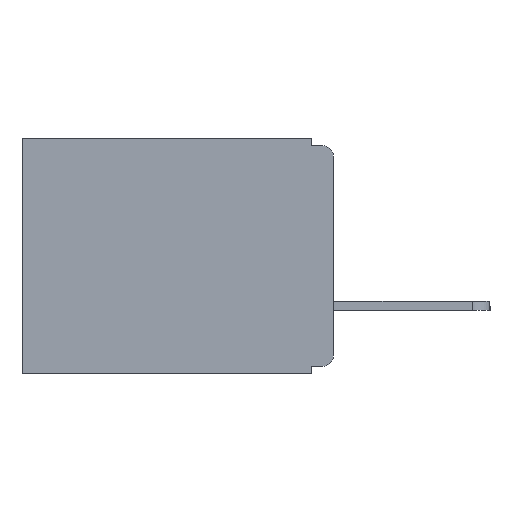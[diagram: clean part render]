
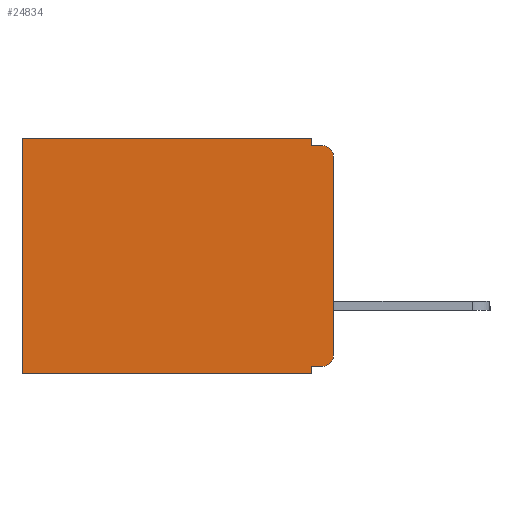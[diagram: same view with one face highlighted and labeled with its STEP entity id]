
A CAD part, left-side view. The second image highlights one B-rep face of the part: STEP entity #24834.
In plain terms, the highlighted planar face has unit normal (-1, 0, 0).
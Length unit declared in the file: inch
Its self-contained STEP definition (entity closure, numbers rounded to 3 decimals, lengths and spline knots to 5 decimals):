
#348 = EDGE_LOOP ( 'NONE', ( #8116, #9659, #23048, #16665, #27672, #12889, #12502, #18715, #5621, #6374 ) ) ;
#965 = EDGE_CURVE ( 'NONE', #14037, #2807, #26319, .T. ) ;
#1911 = VERTEX_POINT ( 'NONE', #20017 ) ;
#2025 = CARTESIAN_POINT ( 'NONE',  ( 0.3, 0.031, 0. ) ) ;
#2807 = VERTEX_POINT ( 'NONE', #31010 ) ;
#3529 = LINE ( 'NONE', #29096, #9255 ) ;
#3638 = VECTOR ( 'NONE', #30112, 39.37008 ) ;
#3853 = VECTOR ( 'NONE', #30522, 39.37008 ) ;
#4380 = EDGE_CURVE ( 'NONE', #2807, #25209, #14804, .T. ) ;
#4521 = DIRECTION ( 'NONE',  ( 1., 0., 0. ) ) ;
#5217 = CARTESIAN_POINT ( 'NONE',  ( 0.3, 0., -0.025 ) ) ;
#5401 = CARTESIAN_POINT ( 'NONE',  ( 0.3, 0., -0.32 ) ) ;
#5452 = EDGE_CURVE ( 'NONE', #5602, #23584, #20508, .T. ) ;
#5579 = EDGE_CURVE ( 'NONE', #1911, #7438, #26923, .T. ) ;
#5602 = VERTEX_POINT ( 'NONE', #27760 ) ;
#5621 = ORIENTED_EDGE ( 'NONE', *, *, #24429, .F. ) ;
#5715 = AXIS2_PLACEMENT_3D ( 'NONE', #19212, #4521, #21662 ) ;
#6340 = CARTESIAN_POINT ( 'NONE',  ( 0.3, 0., -0.33 ) ) ;
#6374 = ORIENTED_EDGE ( 'NONE', *, *, #7396, .T. ) ;
#6567 = CIRCLE ( 'NONE', #19662, 0.015 ) ;
#6825 = VECTOR ( 'NONE', #17000, 39.37008 ) ;
#7396 = EDGE_CURVE ( 'NONE', #10517, #30683, #16577, .T. ) ;
#7438 = VERTEX_POINT ( 'NONE', #13631 ) ;
#7492 = VECTOR ( 'NONE', #14709, 39.37008 ) ;
#7921 = LINE ( 'NONE', #5401, #13666 ) ;
#8116 = ORIENTED_EDGE ( 'NONE', *, *, #12113, .F. ) ;
#8839 = DIRECTION ( 'NONE',  ( 0., 0., -1. ) ) ;
#9255 = VECTOR ( 'NONE', #9646, 39.37008 ) ;
#9421 = CARTESIAN_POINT ( 'NONE',  ( 0.3, 0.031, -0.33 ) ) ;
#9646 = DIRECTION ( 'NONE',  ( 0., 1., 0. ) ) ;
#9659 = ORIENTED_EDGE ( 'NONE', *, *, #21471, .T. ) ;
#10452 = VECTOR ( 'NONE', #8839, 39.37008 ) ;
#10517 = VERTEX_POINT ( 'NONE', #14338 ) ;
#11973 = DIRECTION ( 'NONE',  ( -1., 0., 0. ) ) ;
#12113 = EDGE_CURVE ( 'NONE', #13126, #30683, #29069, .T. ) ;
#12502 = ORIENTED_EDGE ( 'NONE', *, *, #26670, .F. ) ;
#12889 = ORIENTED_EDGE ( 'NONE', *, *, #5579, .T. ) ;
#13126 = VERTEX_POINT ( 'NONE', #5217 ) ;
#13631 = CARTESIAN_POINT ( 'NONE',  ( 0.3, 0.437, -0.33 ) ) ;
#13666 = VECTOR ( 'NONE', #15305, 39.37008 ) ;
#13991 = VECTOR ( 'NONE', #26331, 39.37008 ) ;
#14037 = VERTEX_POINT ( 'NONE', #2025 ) ;
#14094 = DIRECTION ( 'NONE',  ( 0., 0., -1. ) ) ;
#14102 = DIRECTION ( 'NONE',  ( -1., 0., 0. ) ) ;
#14126 = CARTESIAN_POINT ( 'NONE',  ( 0.3, 0.015, -0.305 ) ) ;
#14300 = PLANE ( 'NONE',  #5715 ) ;
#14338 = CARTESIAN_POINT ( 'NONE',  ( 0.3, 0.015, -0.32 ) ) ;
#14709 = DIRECTION ( 'NONE',  ( 0., -1., 0. ) ) ;
#14804 = LINE ( 'NONE', #26223, #7492 ) ;
#15305 = DIRECTION ( 'NONE',  ( 0., 1., 0. ) ) ;
#16577 = CIRCLE ( 'NONE', #19570, 0.015 ) ;
#16665 = ORIENTED_EDGE ( 'NONE', *, *, #965, .F. ) ;
#16728 = CARTESIAN_POINT ( 'NONE',  ( 0.3, 0.031, 0. ) ) ;
#16903 = LINE ( 'NONE', #28135, #3853 ) ;
#17000 = DIRECTION ( 'NONE',  ( 0., 0., -1. ) ) ;
#18292 = CARTESIAN_POINT ( 'NONE',  ( 0.3, 0.031, -0.33 ) ) ;
#18715 = ORIENTED_EDGE ( 'NONE', *, *, #5452, .F. ) ;
#19212 = CARTESIAN_POINT ( 'NONE',  ( 0.3, 0., -0.33 ) ) ;
#19503 = CARTESIAN_POINT ( 'NONE',  ( 0.3, 0., -0.305 ) ) ;
#19570 = AXIS2_PLACEMENT_3D ( 'NONE', #14126, #14102, #14094 ) ;
#19662 = AXIS2_PLACEMENT_3D ( 'NONE', #26553, #11973, #28958 ) ;
#20017 = CARTESIAN_POINT ( 'NONE',  ( 0.3, 0.437, 0. ) ) ;
#20152 = FACE_OUTER_BOUND ( 'NONE', #348, .T. ) ;
#20508 = LINE ( 'NONE', #18292, #13991 ) ;
#20849 = EDGE_CURVE ( 'NONE', #14037, #1911, #3529, .T. ) ;
#21224 = CARTESIAN_POINT ( 'NONE',  ( 0.3, 0.015, -0.01 ) ) ;
#21471 = EDGE_CURVE ( 'NONE', #13126, #25209, #6567, .T. ) ;
#21662 = DIRECTION ( 'NONE',  ( 0., 0., -1. ) ) ;
#23048 = ORIENTED_EDGE ( 'NONE', *, *, #4380, .F. ) ;
#23584 = VERTEX_POINT ( 'NONE', #9421 ) ;
#24429 = EDGE_CURVE ( 'NONE', #10517, #5602, #7921, .T. ) ;
#24834 = ADVANCED_FACE ( 'NONE', ( #20152 ), #14300, .F. ) ;
#25209 = VERTEX_POINT ( 'NONE', #21224 ) ;
#26223 = CARTESIAN_POINT ( 'NONE',  ( 0.3, 0., -0.01 ) ) ;
#26319 = LINE ( 'NONE', #16728, #6825 ) ;
#26331 = DIRECTION ( 'NONE',  ( 0., 0., -1. ) ) ;
#26553 = CARTESIAN_POINT ( 'NONE',  ( 0.3, 0.015, -0.025 ) ) ;
#26670 = EDGE_CURVE ( 'NONE', #23584, #7438, #16903, .T. ) ;
#26923 = LINE ( 'NONE', #29405, #3638 ) ;
#27672 = ORIENTED_EDGE ( 'NONE', *, *, #20849, .T. ) ;
#27760 = CARTESIAN_POINT ( 'NONE',  ( 0.3, 0.031, -0.32 ) ) ;
#28135 = CARTESIAN_POINT ( 'NONE',  ( 0.3, 0., -0.33 ) ) ;
#28958 = DIRECTION ( 'NONE',  ( 0., 0., -1. ) ) ;
#29069 = LINE ( 'NONE', #6340, #10452 ) ;
#29096 = CARTESIAN_POINT ( 'NONE',  ( 0.3, 0., 0. ) ) ;
#29405 = CARTESIAN_POINT ( 'NONE',  ( 0.3, 0.437, -0.33 ) ) ;
#30112 = DIRECTION ( 'NONE',  ( 0., 0., -1. ) ) ;
#30522 = DIRECTION ( 'NONE',  ( 0., 1., 0. ) ) ;
#30683 = VERTEX_POINT ( 'NONE', #19503 ) ;
#31010 = CARTESIAN_POINT ( 'NONE',  ( 0.3, 0.031, -0.01 ) ) ;
